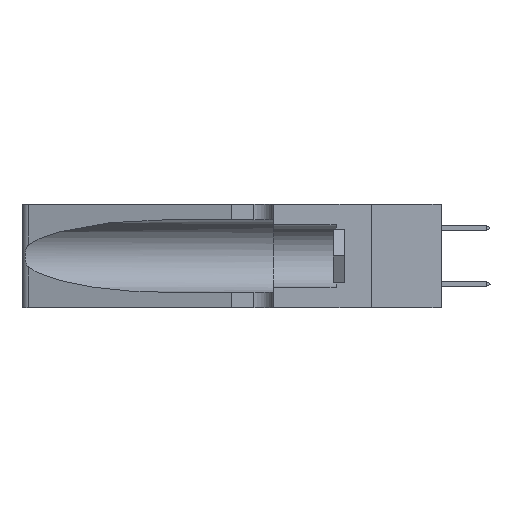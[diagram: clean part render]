
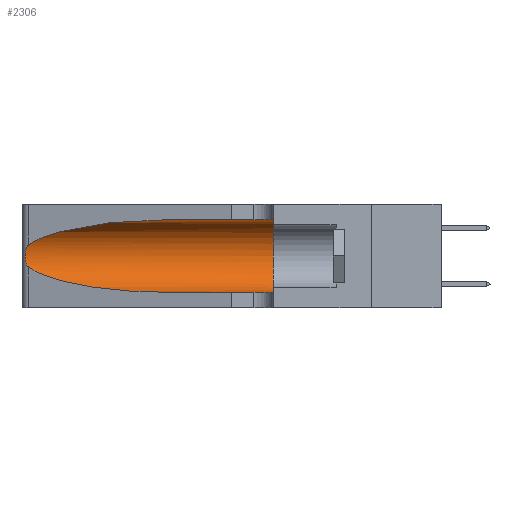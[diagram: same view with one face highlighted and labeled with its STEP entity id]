
A CAD part, left-side view. The second image highlights one B-rep face of the part: STEP entity #2306.
In plain terms, the highlighted cylindrical face has radius 3.308 mm (diameter 6.617 mm), a partial arc.
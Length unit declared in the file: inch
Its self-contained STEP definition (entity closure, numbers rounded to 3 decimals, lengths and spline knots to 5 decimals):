
#133 = DIRECTION ( 'NONE',  ( 0., 1., 0. ) ) ;
#339 = EDGE_LOOP ( 'NONE', ( #2949, #8202, #803, #3646, #10011, #6565 ) ) ;
#570 = CARTESIAN_POINT ( 'NONE',  ( 0.25555, 1.22994, 0.2215 ) ) ;
#638 = EDGE_CURVE ( 'NONE', #11165, #19477, #6502, .T. ) ;
#803 = ORIENTED_EDGE ( 'NONE', *, *, #5914, .T. ) ;
#1038 = EDGE_CURVE ( 'NONE', #8402, #14916, #18954, .T. ) ;
#2071 = CARTESIAN_POINT ( 'NONE',  ( 0.25639, 1.23184, 0.21858 ) ) ;
#2091 = CARTESIAN_POINT ( 'NONE',  ( 0.1305, 1.61858, 0.31525 ) ) ;
#2165 = VECTOR ( 'NONE', #5779, 39.37008 ) ;
#2306 = ADVANCED_FACE ( 'NONE', ( #9528 ), #16853, .F. ) ;
#2441 = VECTOR ( 'NONE', #9494, 39.37008 ) ;
#2752 = CARTESIAN_POINT ( 'NONE',  ( 0.26075, 1.23896, 0.19203 ) ) ;
#2949 = ORIENTED_EDGE ( 'NONE', *, *, #1038, .T. ) ;
#3646 = ORIENTED_EDGE ( 'NONE', *, *, #12619, .T. ) ;
#4097 = CARTESIAN_POINT ( 'NONE',  ( 0.25787, 1.23484, 0.2124 ) ) ;
#4421 = CARTESIAN_POINT ( 'NONE',  ( 0.25789, 1.23486, 0.15765 ) ) ;
#5430 = CARTESIAN_POINT ( 'NONE',  ( 0.25487, 1.22718, 0.14631 ) ) ;
#5438 = CARTESIAN_POINT ( 'NONE',  ( 0.1305, 0.72297, 0.05475 ) ) ;
#5766 = CARTESIAN_POINT ( 'NONE',  ( 0.25639, 1.23186, 0.15144 ) ) ;
#5779 = DIRECTION ( 'NONE',  ( 0., -1., 0. ) ) ;
#5796 = CARTESIAN_POINT ( 'NONE',  ( 0.1305, 1.61858, 0.185 ) ) ;
#5914 = EDGE_CURVE ( 'NONE', #8716, #16661, #12179, .T. ) ;
#6389 = EDGE_CURVE ( 'NONE', #8402, #11165, #16194, .T. ) ;
#6502 = CIRCLE ( 'NONE', #15677, 0.13025 ) ;
#6565 = ORIENTED_EDGE ( 'NONE', *, *, #6389, .F. ) ;
#6976 = CARTESIAN_POINT ( 'NONE',  ( 0.2373, 1.15595, 0.08982 ) ) ;
#8202 = ORIENTED_EDGE ( 'NONE', *, *, #12777, .T. ) ;
#8402 = VERTEX_POINT ( 'NONE', #13690 ) ;
#8716 = VERTEX_POINT ( 'NONE', #14482 ) ;
#8840 = CARTESIAN_POINT ( 'NONE',  ( 0.26018, 1.23835, 0.19895 ) ) ;
#9020 = CARTESIAN_POINT ( 'NONE',  ( 0.1305, 0.72297, 0.31525 ) ) ;
#9494 = DIRECTION ( 'NONE',  ( 0., -1., 0. ) ) ;
#9528 = FACE_OUTER_BOUND ( 'NONE', #339, .T. ) ;
#10011 = ORIENTED_EDGE ( 'NONE', *, *, #638, .F. ) ;
#10710 = DIRECTION ( 'NONE',  ( 0., 0., 1. ) ) ;
#11165 = VERTEX_POINT ( 'NONE', #15220 ) ;
#11651 = CARTESIAN_POINT ( 'NONE',  ( 0.25487, 1.22718, 0.22369 ) ) ;
#11935 = DIRECTION ( 'NONE',  ( 0., -1., 0. ) ) ;
#12179 =( BOUNDED_CURVE ( )  B_SPLINE_CURVE ( 3, ( #5430, #6976, #13051, #17298 ),
 .UNSPECIFIED., .F., .F. ) 
 B_SPLINE_CURVE_WITH_KNOTS ( ( 4, 4 ),
 ( 3.44316, 4.71239 ),
 .UNSPECIFIED. ) 
 CURVE ( )  GEOMETRIC_REPRESENTATION_ITEM ( )  RATIONAL_B_SPLINE_CURVE ( ( 1., 0.87, 0.87, 1. ) ) 
 REPRESENTATION_ITEM ( '' )  );
#12406 = AXIS2_PLACEMENT_3D ( 'NONE', #5796, #11935, #16374 ) ;
#12619 = EDGE_CURVE ( 'NONE', #16661, #19477, #19529, .T. ) ;
#12719 = CARTESIAN_POINT ( 'NONE',  ( 0.25854, 1.2359, 0.20912 ) ) ;
#12777 = EDGE_CURVE ( 'NONE', #14916, #8716, #16537, .T. ) ;
#13051 = CARTESIAN_POINT ( 'NONE',  ( 0.18966, 0.96281, 0.05475 ) ) ;
#13690 = CARTESIAN_POINT ( 'NONE',  ( 0.1305, 0.72297, 0.31525 ) ) ;
#14034 = CARTESIAN_POINT ( 'NONE',  ( 0.1305, 0.35, 0.05475 ) ) ;
#14482 = CARTESIAN_POINT ( 'NONE',  ( 0.25487, 1.22718, 0.14631 ) ) ;
#14916 = VERTEX_POINT ( 'NONE', #19510 ) ;
#15073 = CARTESIAN_POINT ( 'NONE',  ( 0.18966, 0.96281, 0.31525 ) ) ;
#15220 = CARTESIAN_POINT ( 'NONE',  ( 0.1305, 0.35, 0.31525 ) ) ;
#15420 = CARTESIAN_POINT ( 'NONE',  ( 0.1305, 1.61858, 0.05475 ) ) ;
#15677 = AXIS2_PLACEMENT_3D ( 'NONE', #16573, #133, #10710 ) ;
#16194 = LINE ( 'NONE', #2091, #2165 ) ;
#16374 = DIRECTION ( 'NONE',  ( 0., 0., -1. ) ) ;
#16412 = CARTESIAN_POINT ( 'NONE',  ( 0.25856, 1.23593, 0.16098 ) ) ;
#16534 = CARTESIAN_POINT ( 'NONE',  ( 0.26075, 1.23896, 0.178 ) ) ;
#16537 = B_SPLINE_CURVE_WITH_KNOTS ( 'NONE', 3,
 ( #11651, #570, #2071, #4097, #12719, #8840, #2752, #16534, #19453, #16412, #4421, #5766, #18075, #18004 ),
 .UNSPECIFIED., .F., .F.,
 ( 4, 2, 2, 2, 2, 2, 4 ),
 ( 0., 0.00027, 0.00053, 0.00107, 0.0016, 0.00187, 0.00214 ),
 .UNSPECIFIED. ) ;
#16573 = CARTESIAN_POINT ( 'NONE',  ( 0.1305, 0.35, 0.185 ) ) ;
#16661 = VERTEX_POINT ( 'NONE', #5438 ) ;
#16853 = CYLINDRICAL_SURFACE ( 'NONE', #12406, 0.13025 ) ;
#17298 = CARTESIAN_POINT ( 'NONE',  ( 0.1305, 0.72297, 0.05475 ) ) ;
#18004 = CARTESIAN_POINT ( 'NONE',  ( 0.25487, 1.22718, 0.14631 ) ) ;
#18075 = CARTESIAN_POINT ( 'NONE',  ( 0.25555, 1.22993, 0.14849 ) ) ;
#18954 =( BOUNDED_CURVE ( )  B_SPLINE_CURVE ( 3, ( #9020, #15073, #19587, #19646 ),
 .UNSPECIFIED., .F., .F. ) 
 B_SPLINE_CURVE_WITH_KNOTS ( ( 4, 4 ),
 ( 1.5708, 2.84003 ),
 .UNSPECIFIED. ) 
 CURVE ( )  GEOMETRIC_REPRESENTATION_ITEM ( )  RATIONAL_B_SPLINE_CURVE ( ( 1., 0.87, 0.87, 1. ) ) 
 REPRESENTATION_ITEM ( '' )  );
#19453 = CARTESIAN_POINT ( 'NONE',  ( 0.26017, 1.23833, 0.17102 ) ) ;
#19477 = VERTEX_POINT ( 'NONE', #14034 ) ;
#19510 = CARTESIAN_POINT ( 'NONE',  ( 0.25487, 1.22718, 0.22369 ) ) ;
#19529 = LINE ( 'NONE', #15420, #2441 ) ;
#19587 = CARTESIAN_POINT ( 'NONE',  ( 0.2373, 1.15595, 0.28018 ) ) ;
#19646 = CARTESIAN_POINT ( 'NONE',  ( 0.25487, 1.22718, 0.22369 ) ) ;
